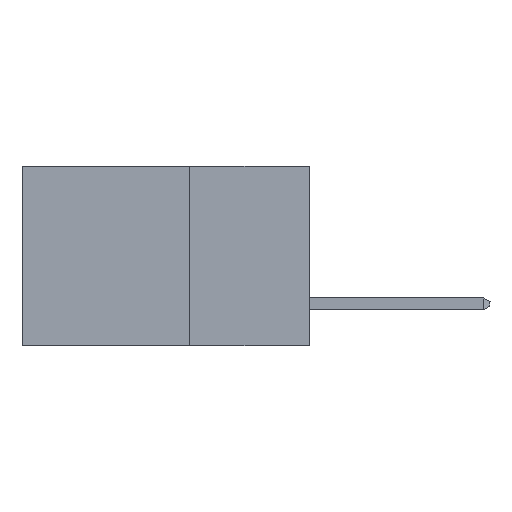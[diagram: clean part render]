
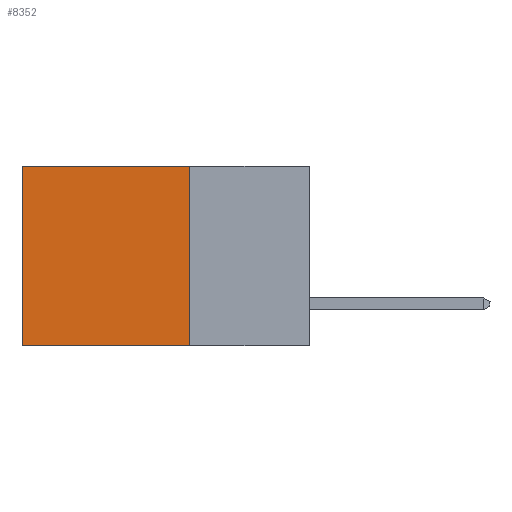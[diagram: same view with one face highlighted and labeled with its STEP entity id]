
A CAD part, left-side view. The second image highlights one B-rep face of the part: STEP entity #8352.
In plain terms, the highlighted planar face has unit normal (-1, 0, 0).
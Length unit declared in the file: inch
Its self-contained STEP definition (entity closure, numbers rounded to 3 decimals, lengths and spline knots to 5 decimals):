
#269 = CARTESIAN_POINT ( 'NONE',  ( 0.2875, 0.6, -0.375 ) ) ;
#737 = DIRECTION ( 'NONE',  ( 1., 0., 0. ) ) ;
#783 = DIRECTION ( 'NONE',  ( 0., 1., 0. ) ) ;
#1067 = EDGE_CURVE ( 'NONE', #3408, #7230, #2362, .T. ) ;
#1129 = LINE ( 'NONE', #5990, #4635 ) ;
#1220 = CARTESIAN_POINT ( 'NONE',  ( 0.2875, 0.25, -0.375 ) ) ;
#1430 = CARTESIAN_POINT ( 'NONE',  ( 0.2875, 0.25, -0.375 ) ) ;
#1458 = EDGE_LOOP ( 'NONE', ( #5140, #6699, #7489, #2845 ) ) ;
#1903 = CARTESIAN_POINT ( 'NONE',  ( 0.2875, 0.25, -0.375 ) ) ;
#1957 = VERTEX_POINT ( 'NONE', #7088 ) ;
#1966 = EDGE_CURVE ( 'NONE', #6698, #3408, #8296, .T. ) ;
#2151 = DIRECTION ( 'NONE',  ( 0., 0., -1. ) ) ;
#2362 = LINE ( 'NONE', #2708, #7080 ) ;
#2708 = CARTESIAN_POINT ( 'NONE',  ( 0.2875, 0.25, -0.375 ) ) ;
#2845 = ORIENTED_EDGE ( 'NONE', *, *, #3021, .T. ) ;
#3012 = FACE_OUTER_BOUND ( 'NONE', #1458, .T. ) ;
#3021 = EDGE_CURVE ( 'NONE', #6698, #1957, #6758, .T. ) ;
#3194 = EDGE_CURVE ( 'NONE', #1957, #7230, #1129, .T. ) ;
#3404 = CARTESIAN_POINT ( 'NONE',  ( 0.2875, 0.25, 0. ) ) ;
#3408 = VERTEX_POINT ( 'NONE', #1220 ) ;
#4635 = VECTOR ( 'NONE', #2151, 39.37008 ) ;
#4739 = VECTOR ( 'NONE', #7626, 39.37008 ) ;
#5140 = ORIENTED_EDGE ( 'NONE', *, *, #3194, .T. ) ;
#5241 = AXIS2_PLACEMENT_3D ( 'NONE', #1430, #737, #6625 ) ;
#5615 = CARTESIAN_POINT ( 'NONE',  ( 0.2875, 0.25, 0. ) ) ;
#5942 = PLANE ( 'NONE',  #5241 ) ;
#5990 = CARTESIAN_POINT ( 'NONE',  ( 0.2875, 0.6, -0.375 ) ) ;
#6358 = VECTOR ( 'NONE', #6554, 39.37008 ) ;
#6554 = DIRECTION ( 'NONE',  ( 0., 0., -1. ) ) ;
#6625 = DIRECTION ( 'NONE',  ( 0., 0., -1. ) ) ;
#6698 = VERTEX_POINT ( 'NONE', #3404 ) ;
#6699 = ORIENTED_EDGE ( 'NONE', *, *, #1067, .F. ) ;
#6758 = LINE ( 'NONE', #5615, #4739 ) ;
#7080 = VECTOR ( 'NONE', #783, 39.37008 ) ;
#7088 = CARTESIAN_POINT ( 'NONE',  ( 0.2875, 0.6, 0. ) ) ;
#7230 = VERTEX_POINT ( 'NONE', #269 ) ;
#7489 = ORIENTED_EDGE ( 'NONE', *, *, #1966, .F. ) ;
#7626 = DIRECTION ( 'NONE',  ( 0., 1., 0. ) ) ;
#8296 = LINE ( 'NONE', #1903, #6358 ) ;
#8352 = ADVANCED_FACE ( 'NONE', ( #3012 ), #5942, .F. ) ;
